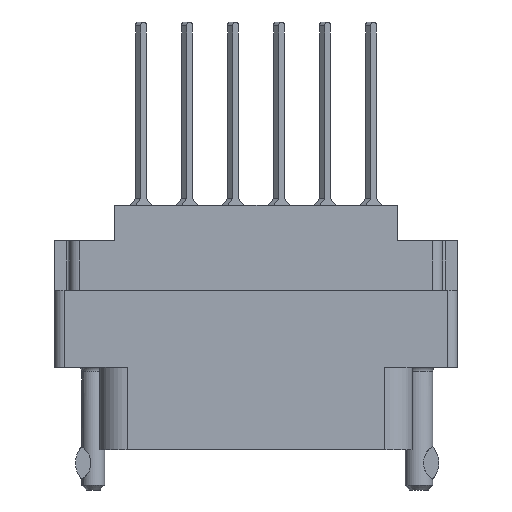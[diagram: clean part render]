
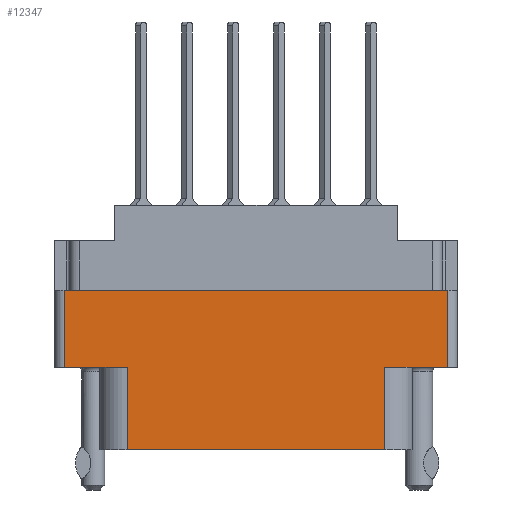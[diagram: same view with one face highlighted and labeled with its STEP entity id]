
A CAD part, front view. The second image highlights one B-rep face of the part: STEP entity #12347.
In plain terms, the highlighted planar face has unit normal (0, -1, 0).
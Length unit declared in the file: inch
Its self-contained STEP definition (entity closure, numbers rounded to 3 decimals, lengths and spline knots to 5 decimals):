
#332 = CARTESIAN_POINT ( 'NONE',  ( 0., -0.343, -0.529 ) ) ;
#478 = VERTEX_POINT ( 'NONE', #4561 ) ;
#1373 = DIRECTION ( 'NONE',  ( 0., 0., -1. ) ) ;
#1967 = VECTOR ( 'NONE', #18708, 39.37008 ) ;
#2032 = EDGE_CURVE ( 'NONE', #7054, #28268, #8058, .T. ) ;
#2580 = VECTOR ( 'NONE', #15218, 39.37008 ) ;
#2838 = EDGE_CURVE ( 'NONE', #22458, #22251, #17800, .T. ) ;
#3174 = CARTESIAN_POINT ( 'NONE',  ( -0.624, -0.343, -0.798 ) ) ;
#3386 = LINE ( 'NONE', #29953, #2580 ) ;
#4224 = CARTESIAN_POINT ( 'NONE',  ( -0.42, -0.343, -0.529 ) ) ;
#4309 = EDGE_CURVE ( 'NONE', #22458, #4838, #28238, .T. ) ;
#4397 = CARTESIAN_POINT ( 'NONE',  ( -0.656, -0.343, -0.277 ) ) ;
#4561 = CARTESIAN_POINT ( 'NONE',  ( -0.624, -0.343, -0.529 ) ) ;
#4838 = VERTEX_POINT ( 'NONE', #25582 ) ;
#5025 = ORIENTED_EDGE ( 'NONE', *, *, #14304, .T. ) ;
#5228 = CARTESIAN_POINT ( 'NONE',  ( 0.624, -0.343, -0.529 ) ) ;
#5412 = VECTOR ( 'NONE', #15457, 39.37008 ) ;
#6365 = FACE_OUTER_BOUND ( 'NONE', #14505, .T. ) ;
#6736 = CARTESIAN_POINT ( 'NONE',  ( 0.42, -0.343, -0.529 ) ) ;
#7016 = LINE ( 'NONE', #26450, #17526 ) ;
#7025 = DIRECTION ( 'NONE',  ( 0., 0., -1. ) ) ;
#7054 = VERTEX_POINT ( 'NONE', #4224 ) ;
#8058 = LINE ( 'NONE', #25008, #18979 ) ;
#8592 = PLANE ( 'NONE',  #21905 ) ;
#9607 = DIRECTION ( 'NONE',  ( 1., 0., 0. ) ) ;
#10097 = CARTESIAN_POINT ( 'NONE',  ( -0.42, -0.343, -0.798 ) ) ;
#12299 = LINE ( 'NONE', #17843, #5412 ) ;
#12342 = EDGE_CURVE ( 'NONE', #22251, #32969, #17700, .T. ) ;
#12347 = ADVANCED_FACE ( 'NONE', ( #6365 ), #8592, .T. ) ;
#13559 = DIRECTION ( 'NONE',  ( 0., 0., 1. ) ) ;
#14304 = EDGE_CURVE ( 'NONE', #478, #7054, #12299, .T. ) ;
#14505 = EDGE_LOOP ( 'NONE', ( #28838, #23525, #28410, #28438, #21533, #14879, #21925, #5025 ) ) ;
#14684 = EDGE_CURVE ( 'NONE', #28268, #32969, #3386, .T. ) ;
#14879 = ORIENTED_EDGE ( 'NONE', *, *, #28707, .F. ) ;
#15218 = DIRECTION ( 'NONE',  ( 1., 0., 0. ) ) ;
#15457 = DIRECTION ( 'NONE',  ( 1., 0., 0. ) ) ;
#17526 = VECTOR ( 'NONE', #13559, 39.37008 ) ;
#17700 = LINE ( 'NONE', #31007, #31863 ) ;
#17800 = LINE ( 'NONE', #332, #19395 ) ;
#17843 = CARTESIAN_POINT ( 'NONE',  ( 0., -0.343, -0.529 ) ) ;
#18520 = DIRECTION ( 'NONE',  ( 0., -1., 0. ) ) ;
#18708 = DIRECTION ( 'NONE',  ( 0., 0., 1. ) ) ;
#18979 = VECTOR ( 'NONE', #7025, 39.37008 ) ;
#19395 = VECTOR ( 'NONE', #28914, 39.37008 ) ;
#21533 = ORIENTED_EDGE ( 'NONE', *, *, #4309, .T. ) ;
#21905 = AXIS2_PLACEMENT_3D ( 'NONE', #3174, #18520, #1373 ) ;
#21925 = ORIENTED_EDGE ( 'NONE', *, *, #24063, .F. ) ;
#22251 = VERTEX_POINT ( 'NONE', #6736 ) ;
#22458 = VERTEX_POINT ( 'NONE', #5228 ) ;
#23525 = ORIENTED_EDGE ( 'NONE', *, *, #14684, .T. ) ;
#23838 = DIRECTION ( 'NONE',  ( 0., 0., -1. ) ) ;
#24063 = EDGE_CURVE ( 'NONE', #478, #26834, #7016, .T. ) ;
#25008 = CARTESIAN_POINT ( 'NONE',  ( -0.42, -0.343, -0.529 ) ) ;
#25582 = CARTESIAN_POINT ( 'NONE',  ( 0.624, -0.343, -0.277 ) ) ;
#26303 = CARTESIAN_POINT ( 'NONE',  ( 0.624, -0.343, -0.798 ) ) ;
#26450 = CARTESIAN_POINT ( 'NONE',  ( -0.624, -0.343, -0.798 ) ) ;
#26834 = VERTEX_POINT ( 'NONE', #32298 ) ;
#27170 = LINE ( 'NONE', #4397, #28407 ) ;
#28238 = LINE ( 'NONE', #26303, #1967 ) ;
#28268 = VERTEX_POINT ( 'NONE', #10097 ) ;
#28407 = VECTOR ( 'NONE', #9607, 39.37008 ) ;
#28410 = ORIENTED_EDGE ( 'NONE', *, *, #12342, .F. ) ;
#28438 = ORIENTED_EDGE ( 'NONE', *, *, #2838, .F. ) ;
#28651 = CARTESIAN_POINT ( 'NONE',  ( 0.42, -0.343, -0.798 ) ) ;
#28707 = EDGE_CURVE ( 'NONE', #26834, #4838, #27170, .T. ) ;
#28838 = ORIENTED_EDGE ( 'NONE', *, *, #2032, .T. ) ;
#28914 = DIRECTION ( 'NONE',  ( -1., 0., 0. ) ) ;
#29953 = CARTESIAN_POINT ( 'NONE',  ( -0.624, -0.343, -0.798 ) ) ;
#31007 = CARTESIAN_POINT ( 'NONE',  ( 0.42, -0.343, -0.529 ) ) ;
#31863 = VECTOR ( 'NONE', #23838, 39.37008 ) ;
#32298 = CARTESIAN_POINT ( 'NONE',  ( -0.624, -0.343, -0.277 ) ) ;
#32969 = VERTEX_POINT ( 'NONE', #28651 ) ;
